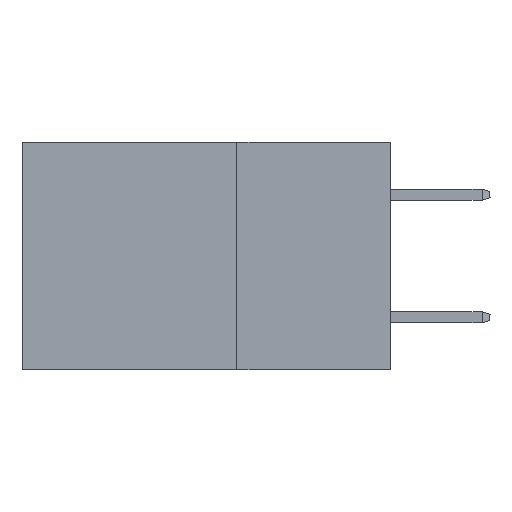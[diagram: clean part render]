
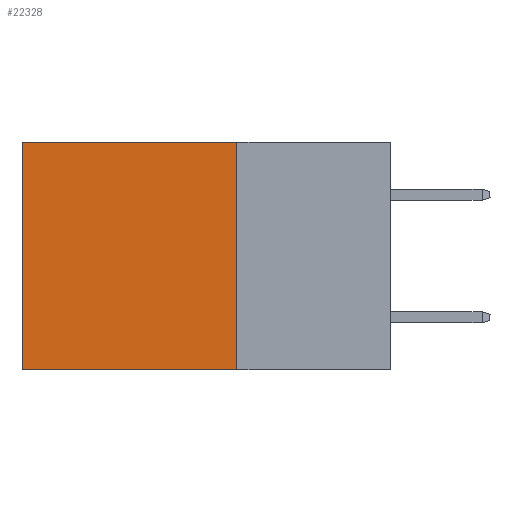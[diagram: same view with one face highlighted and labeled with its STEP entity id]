
A CAD part, left-side view. The second image highlights one B-rep face of the part: STEP entity #22328.
In plain terms, the highlighted planar face has unit normal (-1, 0, 0).
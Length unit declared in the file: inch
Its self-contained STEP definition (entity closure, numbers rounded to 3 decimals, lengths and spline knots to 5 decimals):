
#682 = EDGE_CURVE ( 'NONE', #44829, #26437, #30511, .T. ) ;
#1804 = DIRECTION ( 'NONE',  ( 0., 0., -1. ) ) ;
#4316 = CARTESIAN_POINT ( 'NONE',  ( 0.2875, 0.25, 0. ) ) ;
#4471 = EDGE_CURVE ( 'NONE', #43337, #14131, #16590, .T. ) ;
#4744 = CARTESIAN_POINT ( 'NONE',  ( 0.2875, 0.6, 0. ) ) ;
#6671 = AXIS2_PLACEMENT_3D ( 'NONE', #4316, #32146, #42661 ) ;
#7627 = CARTESIAN_POINT ( 'NONE',  ( 0.2875, 0.6, -0.37 ) ) ;
#9781 = CARTESIAN_POINT ( 'NONE',  ( 0.2875, 0.25, 0. ) ) ;
#13500 = DIRECTION ( 'NONE',  ( 0., 0., -1. ) ) ;
#14131 = VERTEX_POINT ( 'NONE', #7627 ) ;
#16035 = CARTESIAN_POINT ( 'NONE',  ( 0.2875, 0.25, -0.37 ) ) ;
#16038 = LINE ( 'NONE', #20406, #26447 ) ;
#16590 = LINE ( 'NONE', #22725, #41194 ) ;
#17528 = EDGE_CURVE ( 'NONE', #44829, #43337, #29941, .T. ) ;
#18410 = VECTOR ( 'NONE', #1804, 39.37008 ) ;
#18589 = ORIENTED_EDGE ( 'NONE', *, *, #682, .T. ) ;
#18760 = DIRECTION ( 'NONE',  ( 0., 1., 0. ) ) ;
#19884 = FACE_OUTER_BOUND ( 'NONE', #21440, .T. ) ;
#20406 = CARTESIAN_POINT ( 'NONE',  ( 0.2875, 0.6, 0. ) ) ;
#21440 = EDGE_LOOP ( 'NONE', ( #23243, #42080, #33751, #18589 ) ) ;
#21539 = DIRECTION ( 'NONE',  ( 0., 1., 0. ) ) ;
#22328 = ADVANCED_FACE ( 'NONE', ( #19884 ), #35343, .F. ) ;
#22725 = CARTESIAN_POINT ( 'NONE',  ( 0.2875, 0.25, -0.37 ) ) ;
#23243 = ORIENTED_EDGE ( 'NONE', *, *, #23329, .T. ) ;
#23329 = EDGE_CURVE ( 'NONE', #26437, #14131, #16038, .T. ) ;
#24526 = CARTESIAN_POINT ( 'NONE',  ( 0.2875, 0.25, 0. ) ) ;
#26437 = VERTEX_POINT ( 'NONE', #4744 ) ;
#26447 = VECTOR ( 'NONE', #13500, 39.37008 ) ;
#27774 = VECTOR ( 'NONE', #21539, 39.37008 ) ;
#29941 = LINE ( 'NONE', #43653, #18410 ) ;
#30511 = LINE ( 'NONE', #9781, #27774 ) ;
#32146 = DIRECTION ( 'NONE',  ( 1., 0., 0. ) ) ;
#33751 = ORIENTED_EDGE ( 'NONE', *, *, #17528, .F. ) ;
#35343 = PLANE ( 'NONE',  #6671 ) ;
#41194 = VECTOR ( 'NONE', #18760, 39.37008 ) ;
#42080 = ORIENTED_EDGE ( 'NONE', *, *, #4471, .F. ) ;
#42661 = DIRECTION ( 'NONE',  ( 0., 0., -1. ) ) ;
#43337 = VERTEX_POINT ( 'NONE', #16035 ) ;
#43653 = CARTESIAN_POINT ( 'NONE',  ( 0.2875, 0.25, 0. ) ) ;
#44829 = VERTEX_POINT ( 'NONE', #24526 ) ;
